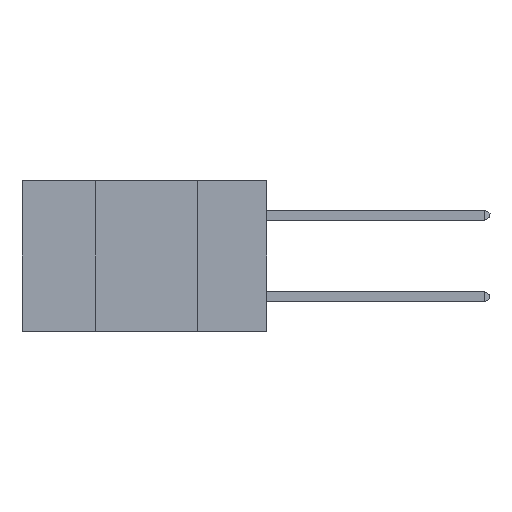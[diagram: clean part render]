
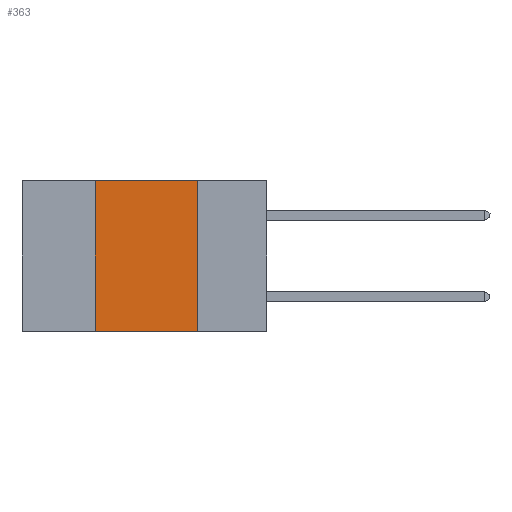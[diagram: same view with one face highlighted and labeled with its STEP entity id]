
A CAD part, left-side view. The second image highlights one B-rep face of the part: STEP entity #363.
In plain terms, the highlighted planar face has unit normal (-1, 0, 0).
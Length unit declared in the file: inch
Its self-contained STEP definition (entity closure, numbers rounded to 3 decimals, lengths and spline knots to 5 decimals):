
#52 = CARTESIAN_POINT ( 'NONE',  ( 0., 0.17, 0. ) ) ;
#133 = DIRECTION ( 'NONE',  ( 0., -1., 0. ) ) ;
#363 = ADVANCED_FACE ( 'NONE', ( #4176 ), #4957, .F. ) ;
#666 = DIRECTION ( 'NONE',  ( 0., 0., 1. ) ) ;
#924 = ORIENTED_EDGE ( 'NONE', *, *, #5506, .F. ) ;
#1031 = CARTESIAN_POINT ( 'NONE',  ( 0., 0.42, -0.37 ) ) ;
#1214 = LINE ( 'NONE', #4534, #4637 ) ;
#2635 = LINE ( 'NONE', #12100, #10974 ) ;
#3088 = ORIENTED_EDGE ( 'NONE', *, *, #4522, .F. ) ;
#3554 = DIRECTION ( 'NONE',  ( 0., 0., -1. ) ) ;
#4176 = FACE_OUTER_BOUND ( 'NONE', #7408, .T. ) ;
#4522 = EDGE_CURVE ( 'NONE', #11969, #7500, #9898, .T. ) ;
#4534 = CARTESIAN_POINT ( 'NONE',  ( 0., 0.6, 0. ) ) ;
#4637 = VECTOR ( 'NONE', #10972, 39.37008 ) ;
#4941 = DIRECTION ( 'NONE',  ( 0., 0., -1. ) ) ;
#4957 = PLANE ( 'NONE',  #5726 ) ;
#5506 = EDGE_CURVE ( 'NONE', #7500, #7889, #1214, .T. ) ;
#5726 = AXIS2_PLACEMENT_3D ( 'NONE', #12179, #6018, #4941 ) ;
#6018 = DIRECTION ( 'NONE',  ( 1., 0., 0. ) ) ;
#6233 = ORIENTED_EDGE ( 'NONE', *, *, #12589, .T. ) ;
#7408 = EDGE_LOOP ( 'NONE', ( #9603, #924, #3088, #6233 ) ) ;
#7413 = CARTESIAN_POINT ( 'NONE',  ( 0., 0.42, 0. ) ) ;
#7500 = VERTEX_POINT ( 'NONE', #13463 ) ;
#7889 = VERTEX_POINT ( 'NONE', #52 ) ;
#7931 = CARTESIAN_POINT ( 'NONE',  ( 0., 0.17, 0. ) ) ;
#9603 = ORIENTED_EDGE ( 'NONE', *, *, #12574, .F. ) ;
#9815 = VERTEX_POINT ( 'NONE', #13786 ) ;
#9898 = LINE ( 'NONE', #7413, #12672 ) ;
#10650 = VECTOR ( 'NONE', #3554, 39.37008 ) ;
#10972 = DIRECTION ( 'NONE',  ( 0., -1., 0. ) ) ;
#10974 = VECTOR ( 'NONE', #133, 39.37008 ) ;
#11969 = VERTEX_POINT ( 'NONE', #1031 ) ;
#12100 = CARTESIAN_POINT ( 'NONE',  ( 0., 0.6, -0.37 ) ) ;
#12179 = CARTESIAN_POINT ( 'NONE',  ( 0., 0.6, 0. ) ) ;
#12574 = EDGE_CURVE ( 'NONE', #7889, #9815, #13473, .T. ) ;
#12589 = EDGE_CURVE ( 'NONE', #11969, #9815, #2635, .T. ) ;
#12672 = VECTOR ( 'NONE', #666, 39.37008 ) ;
#13463 = CARTESIAN_POINT ( 'NONE',  ( 0., 0.42, 0. ) ) ;
#13473 = LINE ( 'NONE', #7931, #10650 ) ;
#13786 = CARTESIAN_POINT ( 'NONE',  ( 0., 0.17, -0.37 ) ) ;
